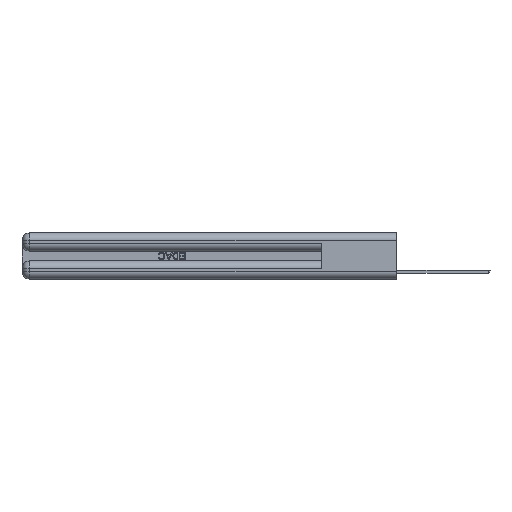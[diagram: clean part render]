
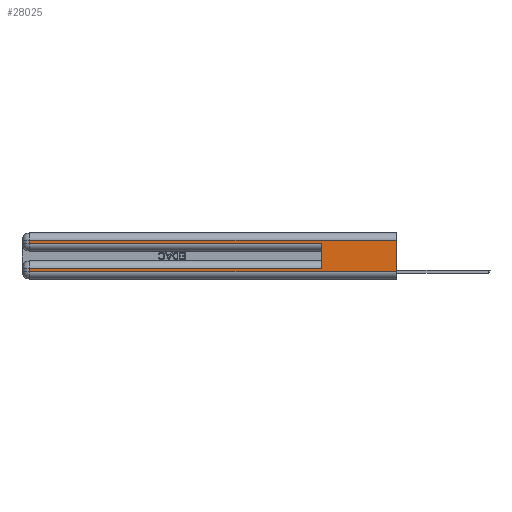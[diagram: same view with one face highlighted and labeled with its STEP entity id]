
A CAD part, left-side view. The second image highlights one B-rep face of the part: STEP entity #28025.
In plain terms, the highlighted planar face has unit normal (-1, 0, 0).
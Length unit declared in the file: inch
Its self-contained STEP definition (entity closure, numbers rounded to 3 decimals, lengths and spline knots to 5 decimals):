
#260 = CARTESIAN_POINT ( 'NONE',  ( 0., 0., 0.31 ) ) ;
#587 = ORIENTED_EDGE ( 'NONE', *, *, #14305, .T. ) ;
#1210 = ORIENTED_EDGE ( 'NONE', *, *, #21001, .T. ) ;
#1246 = LINE ( 'NONE', #27725, #8906 ) ;
#1531 = VECTOR ( 'NONE', #26256, 39.37008 ) ;
#1801 = EDGE_CURVE ( 'NONE', #27891, #17136, #2774, .T. ) ;
#1916 = VECTOR ( 'NONE', #34419, 39.37008 ) ;
#2361 = CARTESIAN_POINT ( 'NONE',  ( 0., 2.94, 0.285 ) ) ;
#2774 = LINE ( 'NONE', #32213, #1531 ) ;
#3723 = CARTESIAN_POINT ( 'NONE',  ( 0., 0., 0.06 ) ) ;
#4196 = CARTESIAN_POINT ( 'NONE',  ( 0., 2.94, 0.085 ) ) ;
#4213 = FACE_OUTER_BOUND ( 'NONE', #17175, .T. ) ;
#4349 = LINE ( 'NONE', #9948, #4491 ) ;
#4491 = VECTOR ( 'NONE', #15403, 39.37008 ) ;
#4553 = ORIENTED_EDGE ( 'NONE', *, *, #1801, .T. ) ;
#4643 = LINE ( 'NONE', #6938, #21328 ) ;
#4980 = LINE ( 'NONE', #23382, #1916 ) ;
#6507 = DIRECTION ( 'NONE',  ( 0., 0., -1. ) ) ;
#6938 = CARTESIAN_POINT ( 'NONE',  ( 0., 0., 0.085 ) ) ;
#7298 = DIRECTION ( 'NONE',  ( 0., 0., -1. ) ) ;
#7478 = LINE ( 'NONE', #23246, #29190 ) ;
#8196 = ORIENTED_EDGE ( 'NONE', *, *, #28907, .T. ) ;
#8689 = VERTEX_POINT ( 'NONE', #28623 ) ;
#8906 = VECTOR ( 'NONE', #25616, 39.37008 ) ;
#9209 = DIRECTION ( 'NONE',  ( 0., -1., 0. ) ) ;
#9634 = CARTESIAN_POINT ( 'NONE',  ( 0., 0.6, 0.085 ) ) ;
#9948 = CARTESIAN_POINT ( 'NONE',  ( 0., 0., 0.06 ) ) ;
#11064 = ORIENTED_EDGE ( 'NONE', *, *, #25337, .F. ) ;
#12443 = PLANE ( 'NONE',  #15134 ) ;
#14305 = EDGE_CURVE ( 'NONE', #8689, #16612, #4349, .T. ) ;
#15134 = AXIS2_PLACEMENT_3D ( 'NONE', #22446, #25606, #6507 ) ;
#15362 = VERTEX_POINT ( 'NONE', #4196 ) ;
#15403 = DIRECTION ( 'NONE',  ( 0., -1., 0. ) ) ;
#16612 = VERTEX_POINT ( 'NONE', #3723 ) ;
#16857 = ORIENTED_EDGE ( 'NONE', *, *, #32316, .T. ) ;
#17136 = VERTEX_POINT ( 'NONE', #28336 ) ;
#17175 = EDGE_LOOP ( 'NONE', ( #20252, #4553, #16857, #1210, #11064, #8196, #20770, #587 ) ) ;
#17292 = EDGE_CURVE ( 'NONE', #15362, #8689, #7478, .T. ) ;
#17644 = DIRECTION ( 'NONE',  ( 0., 1., 0. ) ) ;
#19184 = LINE ( 'NONE', #32308, #23219 ) ;
#19396 = VERTEX_POINT ( 'NONE', #19773 ) ;
#19773 = CARTESIAN_POINT ( 'NONE',  ( 0., 0.6, 0.285 ) ) ;
#20076 = LINE ( 'NONE', #30229, #22106 ) ;
#20252 = ORIENTED_EDGE ( 'NONE', *, *, #21327, .F. ) ;
#20770 = ORIENTED_EDGE ( 'NONE', *, *, #17292, .T. ) ;
#21001 = EDGE_CURVE ( 'NONE', #23238, #19396, #20076, .T. ) ;
#21327 = EDGE_CURVE ( 'NONE', #27891, #16612, #19184, .T. ) ;
#21328 = VECTOR ( 'NONE', #17644, 39.37008 ) ;
#22106 = VECTOR ( 'NONE', #9209, 39.37008 ) ;
#22446 = CARTESIAN_POINT ( 'NONE',  ( 0., 0., 0.37 ) ) ;
#23219 = VECTOR ( 'NONE', #27063, 39.37008 ) ;
#23238 = VERTEX_POINT ( 'NONE', #2361 ) ;
#23246 = CARTESIAN_POINT ( 'NONE',  ( 0., 2.94, 0.37 ) ) ;
#23382 = CARTESIAN_POINT ( 'NONE',  ( 0., 2.94, 0.37 ) ) ;
#25337 = EDGE_CURVE ( 'NONE', #26694, #19396, #1246, .T. ) ;
#25606 = DIRECTION ( 'NONE',  ( 1., 0., 0. ) ) ;
#25616 = DIRECTION ( 'NONE',  ( 0., 0., 1. ) ) ;
#26256 = DIRECTION ( 'NONE',  ( 0., 1., 0. ) ) ;
#26694 = VERTEX_POINT ( 'NONE', #9634 ) ;
#27063 = DIRECTION ( 'NONE',  ( 0., 0., -1. ) ) ;
#27725 = CARTESIAN_POINT ( 'NONE',  ( 0., 0.6, 0.145 ) ) ;
#27891 = VERTEX_POINT ( 'NONE', #260 ) ;
#28025 = ADVANCED_FACE ( 'NONE', ( #4213 ), #12443, .F. ) ;
#28336 = CARTESIAN_POINT ( 'NONE',  ( 0., 2.94, 0.31 ) ) ;
#28623 = CARTESIAN_POINT ( 'NONE',  ( 0., 2.94, 0.06 ) ) ;
#28907 = EDGE_CURVE ( 'NONE', #26694, #15362, #4643, .T. ) ;
#29190 = VECTOR ( 'NONE', #7298, 39.37008 ) ;
#30229 = CARTESIAN_POINT ( 'NONE',  ( 0., 0., 0.285 ) ) ;
#32213 = CARTESIAN_POINT ( 'NONE',  ( 0., 0., 0.31 ) ) ;
#32308 = CARTESIAN_POINT ( 'NONE',  ( 0., 0., 0.37 ) ) ;
#32316 = EDGE_CURVE ( 'NONE', #17136, #23238, #4980, .T. ) ;
#34419 = DIRECTION ( 'NONE',  ( 0., 0., -1. ) ) ;
